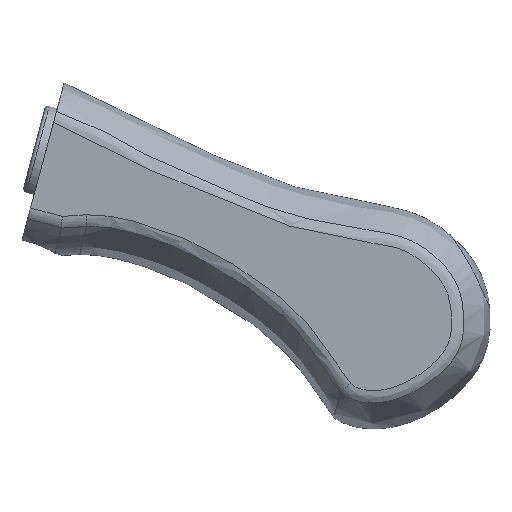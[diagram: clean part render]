
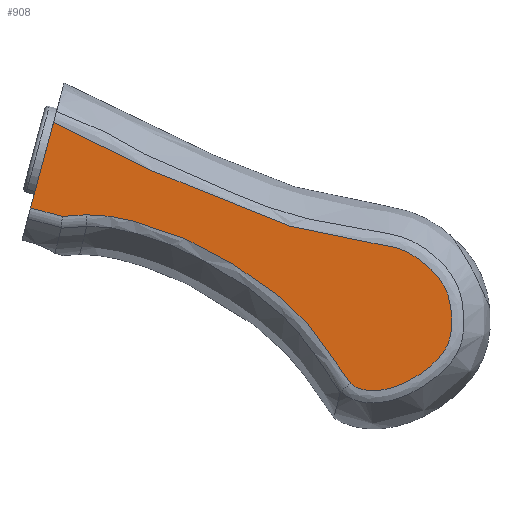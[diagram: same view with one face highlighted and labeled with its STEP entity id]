
A CAD part, left-side view. The second image highlights one B-rep face of the part: STEP entity #908.
In plain terms, the highlighted planar face has unit normal (-1, 0, 0).
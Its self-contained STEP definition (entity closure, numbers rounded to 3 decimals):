
#84=B_SPLINE_CURVE_WITH_KNOTS('',3,(#1878,#1879,#1880,#1881,#1882,#1883,
#1884,#1885,#1886,#1887,#1888,#1889,#1890,#1891,#1892,#1893,#1894,#1895,
#1896,#1897,#1898,#1899,#1900,#1901,#1902,#1903,#1904,#1905,#1906,#1907,
#1908,#1909,#1910,#1911,#1912,#1913,#1914,#1915,#1916,#1917,#1918,#1919),
 .UNSPECIFIED.,.F.,.F.,(4,1,1,1,1,1,1,1,1,1,1,1,1,1,1,1,1,1,1,1,1,1,1,1,
1,1,1,1,1,1,1,1,1,1,1,1,1,1,1,4),(-16.712,-16.607,-16.458,
-16.159,-15.56,-15.261,-14.962,
-14.663,-14.364,-13.167,-11.971,
-11.373,-10.774,-10.176,-9.578,-7.983,
-7.584,-7.185,-6.786,-6.587,
-6.387,-5.988,-5.59,-5.191,
-4.792,-4.593,-4.393,-3.994,
-3.595,-3.396,-3.197,-2.997,
-2.798,-2.399,-1.801,-1.202,
-0.604,-0.305,-0.156,-0.03),
 .UNSPECIFIED.);
#85=B_SPLINE_CURVE_WITH_KNOTS('',3,(#1926,#1927,#1928,#1929,#1930,#1931,
#1932,#1933,#1934,#1935,#1936,#1937,#1938,#1939,#1940,#1941,#1942,#1943,
#1944,#1945,#1946),.UNSPECIFIED.,.F.,.F.,(4,1,1,1,1,1,1,1,1,1,1,1,1,1,1,
1,2,4),(-8.965,-8.106,-7.205,-6.304,
-5.404,-4.503,-3.603,-2.702,
-2.252,-1.801,-1.351,-0.901,
-0.45,-0.225,-0.113,-0.056,
0.,0.012),.UNSPECIFIED.);
#152=FACE_OUTER_BOUND('',#207,.T.);
#207=EDGE_LOOP('',(#672,#673,#674,#675,#676));
#265=LINE('',#1921,#321);
#266=LINE('',#1923,#322);
#267=LINE('',#1925,#323);
#321=VECTOR('',#1088,10.);
#322=VECTOR('',#1089,10.);
#323=VECTOR('',#1090,10.);
#397=VERTEX_POINT('',#1876);
#398=VERTEX_POINT('',#1877);
#399=VERTEX_POINT('',#1920);
#400=VERTEX_POINT('',#1922);
#401=VERTEX_POINT('',#1924);
#502=EDGE_CURVE('',#397,#398,#84,.T.);
#503=EDGE_CURVE('',#399,#397,#265,.T.);
#504=EDGE_CURVE('',#400,#399,#266,.T.);
#505=EDGE_CURVE('',#401,#400,#267,.T.);
#506=EDGE_CURVE('',#398,#401,#85,.T.);
#672=ORIENTED_EDGE('',*,*,#502,.F.);
#673=ORIENTED_EDGE('',*,*,#503,.F.);
#674=ORIENTED_EDGE('',*,*,#504,.F.);
#675=ORIENTED_EDGE('',*,*,#505,.F.);
#676=ORIENTED_EDGE('',*,*,#506,.F.);
#874=PLANE('',#979);
#908=ADVANCED_FACE('',(#152),#874,.T.);
#979=AXIS2_PLACEMENT_3D('',#1875,#1086,#1087);
#1086=DIRECTION('center_axis',(-1.,0.,0.));
#1087=DIRECTION('ref_axis',(0.,-1.,0.));
#1088=DIRECTION('',(0.,-0.259,0.966));
#1089=DIRECTION('',(0.,0.966,0.259));
#1090=DIRECTION('',(0.,0.997,-0.072));
#1875=CARTESIAN_POINT('Origin',(-17.635,-50.656,-29.496));
#1876=CARTESIAN_POINT('',(-17.635,-2.824,7.348));
#1877=CARTESIAN_POINT('',(-17.635,-84.663,-64.467));
#1878=CARTESIAN_POINT('Ctrl Pts',(-17.635,-2.824,7.348));
#1879=CARTESIAN_POINT('Ctrl Pts',(-17.635,-3.146,7.211));
#1880=CARTESIAN_POINT('Ctrl Pts',(-17.635,-3.927,6.883));
#1881=CARTESIAN_POINT('Ctrl Pts',(-17.635,-5.625,6.161));
#1882=CARTESIAN_POINT('Ctrl Pts',(-17.635,-8.839,4.799));
#1883=CARTESIAN_POINT('Ctrl Pts',(-17.635,-12.509,3.24));
#1884=CARTESIAN_POINT('Ctrl Pts',(-17.635,-16.118,1.539));
#1885=CARTESIAN_POINT('Ctrl Pts',(-17.635,-18.753,0.118));
#1886=CARTESIAN_POINT('Ctrl Pts',(-17.635,-21.295,-1.459));
#1887=CARTESIAN_POINT('Ctrl Pts',(-17.635,-26.494,-4.425));
#1888=CARTESIAN_POINT('Ctrl Pts',(-17.635,-34.658,-8.13));
#1889=CARTESIAN_POINT('Ctrl Pts',(-17.635,-43.842,-12.014));
#1890=CARTESIAN_POINT('Ctrl Pts',(-17.635,-51.168,-15.165));
#1891=CARTESIAN_POINT('Ctrl Pts',(-17.635,-56.665,-17.53));
#1892=CARTESIAN_POINT('Ctrl Pts',(-17.635,-62.301,-19.548));
#1893=CARTESIAN_POINT('Ctrl Pts',(-17.635,-71.216,-22.214));
#1894=CARTESIAN_POINT('Ctrl Pts',(-17.635,-79.623,-24.263));
#1895=CARTESIAN_POINT('Ctrl Pts',(-17.635,-87.506,-25.51));
#1896=CARTESIAN_POINT('Ctrl Pts',(-17.635,-91.461,-26.025));
#1897=CARTESIAN_POINT('Ctrl Pts',(-17.635,-94.754,-26.495));
#1898=CARTESIAN_POINT('Ctrl Pts',(-17.635,-97.335,-27.145));
#1899=CARTESIAN_POINT('Ctrl Pts',(-17.635,-99.829,-28.083));
#1900=CARTESIAN_POINT('Ctrl Pts',(-17.635,-102.737,-29.71));
#1901=CARTESIAN_POINT('Ctrl Pts',(-17.635,-105.913,-32.138));
#1902=CARTESIAN_POINT('Ctrl Pts',(-17.635,-108.705,-35.003));
#1903=CARTESIAN_POINT('Ctrl Pts',(-17.635,-110.535,-37.809));
#1904=CARTESIAN_POINT('Ctrl Pts',(-17.635,-111.51,-40.289));
#1905=CARTESIAN_POINT('Ctrl Pts',(-17.635,-112.171,-42.869));
#1906=CARTESIAN_POINT('Ctrl Pts',(-17.635,-112.533,-46.18));
#1907=CARTESIAN_POINT('Ctrl Pts',(-17.635,-112.492,-49.513));
#1908=CARTESIAN_POINT('Ctrl Pts',(-17.635,-112.017,-52.139));
#1909=CARTESIAN_POINT('Ctrl Pts',(-17.635,-111.339,-54.024));
#1910=CARTESIAN_POINT('Ctrl Pts',(-17.635,-110.334,-55.754));
#1911=CARTESIAN_POINT('Ctrl Pts',(-17.635,-108.695,-57.852));
#1912=CARTESIAN_POINT('Ctrl Pts',(-17.635,-105.81,-60.625));
#1913=CARTESIAN_POINT('Ctrl Pts',(-17.635,-101.398,-63.629));
#1914=CARTESIAN_POINT('Ctrl Pts',(-17.635,-95.893,-66.036));
#1915=CARTESIAN_POINT('Ctrl Pts',(-17.635,-90.893,-66.805));
#1916=CARTESIAN_POINT('Ctrl Pts',(-17.635,-87.422,-66.17));
#1917=CARTESIAN_POINT('Ctrl Pts',(-17.635,-85.682,-65.343));
#1918=CARTESIAN_POINT('Ctrl Pts',(-17.635,-84.961,-64.763));
#1919=CARTESIAN_POINT('Ctrl Pts',(-17.635,-84.663,-64.467));
#1920=CARTESIAN_POINT('',(-17.635,3.487,-16.205));
#1921=CARTESIAN_POINT('',(-17.635,3.789,-17.333));
#1922=CARTESIAN_POINT('',(-17.635,-5.254,-18.547));
#1923=CARTESIAN_POINT('',(-17.635,-5.574,-18.633));
#1924=CARTESIAN_POINT('',(-17.635,-11.836,-18.075));
#1925=CARTESIAN_POINT('',(-17.635,-15.79,-17.792));
#1926=CARTESIAN_POINT('Ctrl Pts',(-17.635,-84.663,-64.467));
#1927=CARTESIAN_POINT('Ctrl Pts',(-17.635,-83.049,-62.101));
#1928=CARTESIAN_POINT('Ctrl Pts',(-17.635,-79.783,-57.232));
#1929=CARTESIAN_POINT('Ctrl Pts',(-17.635,-74.648,-49.989));
#1930=CARTESIAN_POINT('Ctrl Pts',(-17.635,-68.454,-43.401));
#1931=CARTESIAN_POINT('Ctrl Pts',(-17.635,-61.474,-37.699));
#1932=CARTESIAN_POINT('Ctrl Pts',(-17.635,-54.009,-32.644));
#1933=CARTESIAN_POINT('Ctrl Pts',(-17.635,-46.219,-28.119));
#1934=CARTESIAN_POINT('Ctrl Pts',(-17.635,-39.493,-24.792));
#1935=CARTESIAN_POINT('Ctrl Pts',(-17.635,-33.907,-22.589));
#1936=CARTESIAN_POINT('Ctrl Pts',(-17.635,-29.619,-21.219));
#1937=CARTESIAN_POINT('Ctrl Pts',(-17.635,-25.304,-19.944));
#1938=CARTESIAN_POINT('Ctrl Pts',(-17.635,-20.919,-18.88));
#1939=CARTESIAN_POINT('Ctrl Pts',(-17.635,-17.203,-18.327));
#1940=CARTESIAN_POINT('Ctrl Pts',(-17.635,-14.587,-18.137));
#1941=CARTESIAN_POINT('Ctrl Pts',(-17.635,-13.272,-18.091));
#1942=CARTESIAN_POINT('Ctrl Pts',(-17.635,-12.519,-18.078));
#1943=CARTESIAN_POINT('Ctrl Pts',(-17.635,-12.144,-18.075));
#1944=CARTESIAN_POINT('Ctrl Pts',(-17.635,-11.916,-18.075));
#1945=CARTESIAN_POINT('Ctrl Pts',(-17.635,-11.876,-18.075));
#1946=CARTESIAN_POINT('Ctrl Pts',(-17.635,-11.836,-18.075));
